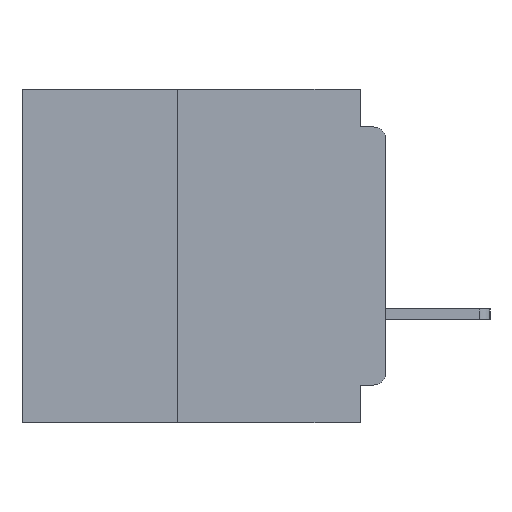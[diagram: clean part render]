
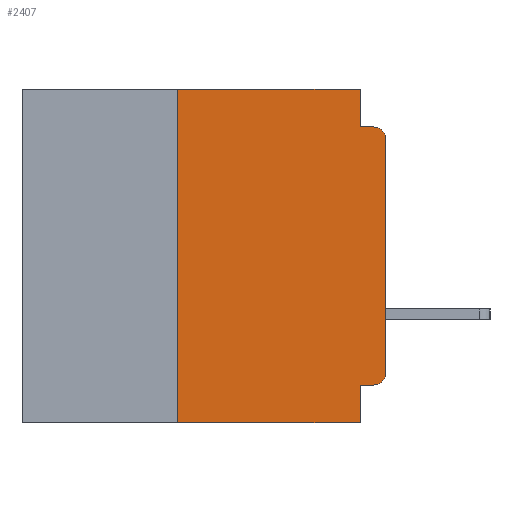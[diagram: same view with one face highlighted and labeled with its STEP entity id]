
A CAD part, left-side view. The second image highlights one B-rep face of the part: STEP entity #2407.
In plain terms, the highlighted planar face has unit normal (-1, 0, 0).
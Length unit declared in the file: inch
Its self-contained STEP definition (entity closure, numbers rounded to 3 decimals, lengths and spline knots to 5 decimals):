
#745 = ORIENTED_EDGE ( 'NONE', *, *, #38674, .F. ) ;
#1903 = DIRECTION ( 'NONE',  ( 0., 0., -1. ) ) ;
#1983 = VECTOR ( 'NONE', #16574, 39.37008 ) ;
#1991 = DIRECTION ( 'NONE',  ( 1., 0., 0. ) ) ;
#2028 = VECTOR ( 'NONE', #36347, 39.37008 ) ;
#2100 = CARTESIAN_POINT ( 'NONE',  ( 0., 0.015, -0.06 ) ) ;
#2135 = CARTESIAN_POINT ( 'NONE',  ( 0., 0.437, 0. ) ) ;
#2275 = CARTESIAN_POINT ( 'NONE',  ( 0., 0., -0.06 ) ) ;
#2407 = ADVANCED_FACE ( 'NONE', ( #24561 ), #2717, .F. ) ;
#2661 = VERTEX_POINT ( 'NONE', #40951 ) ;
#2717 = PLANE ( 'NONE',  #25965 ) ;
#3074 = LINE ( 'NONE', #20625, #2028 ) ;
#3439 = VERTEX_POINT ( 'NONE', #9915 ) ;
#3565 = LINE ( 'NONE', #5092, #27978 ) ;
#3598 = EDGE_CURVE ( 'NONE', #2661, #4166, #3565, .T. ) ;
#4166 = VERTEX_POINT ( 'NONE', #30262 ) ;
#4484 = LINE ( 'NONE', #23151, #26908 ) ;
#5092 = CARTESIAN_POINT ( 'NONE',  ( 0., 0.437, 0. ) ) ;
#5333 = DIRECTION ( 'NONE',  ( 0., 0., -1. ) ) ;
#5709 = EDGE_LOOP ( 'NONE', ( #23992, #15584, #27471, #26052, #34728, #37566, #14525, #10706, #745, #32474 ) ) ;
#5774 = VERTEX_POINT ( 'NONE', #27625 ) ;
#6024 = VERTEX_POINT ( 'NONE', #35799 ) ;
#6410 = EDGE_CURVE ( 'NONE', #9941, #2661, #14553, .T. ) ;
#8575 = EDGE_CURVE ( 'NONE', #4166, #3439, #37599, .T. ) ;
#9915 = CARTESIAN_POINT ( 'NONE',  ( 0., 0.031, -0.045 ) ) ;
#9941 = VERTEX_POINT ( 'NONE', #20162 ) ;
#10145 = LINE ( 'NONE', #37665, #25998 ) ;
#10286 = EDGE_CURVE ( 'NONE', #3439, #12580, #24959, .T. ) ;
#10307 = AXIS2_PLACEMENT_3D ( 'NONE', #2100, #24448, #5333 ) ;
#10706 = ORIENTED_EDGE ( 'NONE', *, *, #39125, .F. ) ;
#11273 = CIRCLE ( 'NONE', #10307, 0.015 ) ;
#12580 = VERTEX_POINT ( 'NONE', #13933 ) ;
#13933 = CARTESIAN_POINT ( 'NONE',  ( 0., 0.015, -0.045 ) ) ;
#14239 = CARTESIAN_POINT ( 'NONE',  ( 0., 0.015, -0.34 ) ) ;
#14525 = ORIENTED_EDGE ( 'NONE', *, *, #41229, .T. ) ;
#14553 = LINE ( 'NONE', #40581, #38787 ) ;
#15584 = ORIENTED_EDGE ( 'NONE', *, *, #30214, .T. ) ;
#15588 = VECTOR ( 'NONE', #18750, 39.37008 ) ;
#15625 = CIRCLE ( 'NONE', #32117, 0.015 ) ;
#16574 = DIRECTION ( 'NONE',  ( 0., 0., -1. ) ) ;
#17431 = DIRECTION ( 'NONE',  ( 0., 0., -1. ) ) ;
#18029 = VERTEX_POINT ( 'NONE', #41123 ) ;
#18510 = DIRECTION ( 'NONE',  ( 0., 0., 1. ) ) ;
#18750 = DIRECTION ( 'NONE',  ( 0., -1., 0. ) ) ;
#20162 = CARTESIAN_POINT ( 'NONE',  ( 0., 0.25, -0.4 ) ) ;
#20625 = CARTESIAN_POINT ( 'NONE',  ( 0., 0., -0.355 ) ) ;
#21063 = DIRECTION ( 'NONE',  ( 0., -1., 0. ) ) ;
#21748 = EDGE_CURVE ( 'NONE', #27280, #6024, #15625, .T. ) ;
#22894 = CARTESIAN_POINT ( 'NONE',  ( 0., 0.031, 0. ) ) ;
#22917 = CARTESIAN_POINT ( 'NONE',  ( 0., 0.031, -0.4 ) ) ;
#23058 = EDGE_CURVE ( 'NONE', #6024, #27812, #10145, .T. ) ;
#23151 = CARTESIAN_POINT ( 'NONE',  ( 0., 0.437, -0.4 ) ) ;
#23992 = ORIENTED_EDGE ( 'NONE', *, *, #23058, .T. ) ;
#24448 = DIRECTION ( 'NONE',  ( -1., 0., 0. ) ) ;
#24561 = FACE_OUTER_BOUND ( 'NONE', #5709, .T. ) ;
#24959 = LINE ( 'NONE', #31319, #15588 ) ;
#25965 = AXIS2_PLACEMENT_3D ( 'NONE', #2135, #1991, #1903 ) ;
#25998 = VECTOR ( 'NONE', #34490, 39.37008 ) ;
#26052 = ORIENTED_EDGE ( 'NONE', *, *, #8575, .F. ) ;
#26293 = DIRECTION ( 'NONE',  ( 0., -1., 0. ) ) ;
#26908 = VECTOR ( 'NONE', #26293, 39.37008 ) ;
#27280 = VERTEX_POINT ( 'NONE', #31473 ) ;
#27471 = ORIENTED_EDGE ( 'NONE', *, *, #10286, .F. ) ;
#27625 = CARTESIAN_POINT ( 'NONE',  ( 0., 0.031, -0.355 ) ) ;
#27812 = VERTEX_POINT ( 'NONE', #2275 ) ;
#27978 = VECTOR ( 'NONE', #21063, 39.37008 ) ;
#29222 = VECTOR ( 'NONE', #32455, 39.37008 ) ;
#30214 = EDGE_CURVE ( 'NONE', #27812, #12580, #11273, .T. ) ;
#30262 = CARTESIAN_POINT ( 'NONE',  ( 0., 0.031, 0. ) ) ;
#31319 = CARTESIAN_POINT ( 'NONE',  ( 0., 0., -0.045 ) ) ;
#31473 = CARTESIAN_POINT ( 'NONE',  ( 0., 0.015, -0.355 ) ) ;
#32117 = AXIS2_PLACEMENT_3D ( 'NONE', #14239, #36355, #17431 ) ;
#32455 = DIRECTION ( 'NONE',  ( 0., 0., -1. ) ) ;
#32474 = ORIENTED_EDGE ( 'NONE', *, *, #21748, .T. ) ;
#34490 = DIRECTION ( 'NONE',  ( 0., 0., 1. ) ) ;
#34728 = ORIENTED_EDGE ( 'NONE', *, *, #3598, .F. ) ;
#34895 = LINE ( 'NONE', #22917, #1983 ) ;
#35799 = CARTESIAN_POINT ( 'NONE',  ( 0., 0., -0.34 ) ) ;
#36347 = DIRECTION ( 'NONE',  ( 0., 1., 0. ) ) ;
#36355 = DIRECTION ( 'NONE',  ( -1., 0., 0. ) ) ;
#37566 = ORIENTED_EDGE ( 'NONE', *, *, #6410, .F. ) ;
#37599 = LINE ( 'NONE', #22894, #29222 ) ;
#37665 = CARTESIAN_POINT ( 'NONE',  ( 0., 0., 0. ) ) ;
#38674 = EDGE_CURVE ( 'NONE', #27280, #5774, #3074, .T. ) ;
#38787 = VECTOR ( 'NONE', #18510, 39.37008 ) ;
#39125 = EDGE_CURVE ( 'NONE', #5774, #18029, #34895, .T. ) ;
#40581 = CARTESIAN_POINT ( 'NONE',  ( 0., 0.25, -0.4 ) ) ;
#40951 = CARTESIAN_POINT ( 'NONE',  ( 0., 0.25, 0. ) ) ;
#41123 = CARTESIAN_POINT ( 'NONE',  ( 0., 0.031, -0.4 ) ) ;
#41229 = EDGE_CURVE ( 'NONE', #9941, #18029, #4484, .T. ) ;
